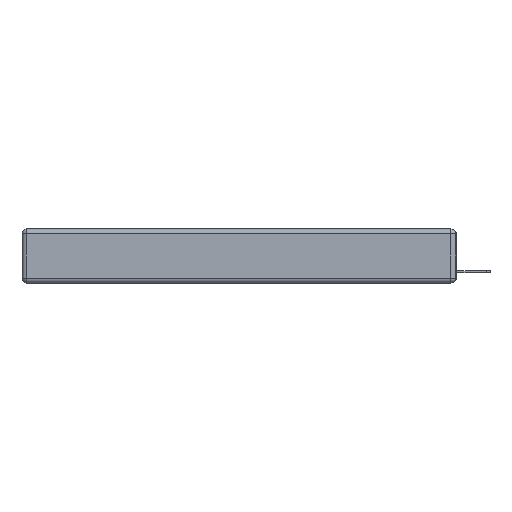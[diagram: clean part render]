
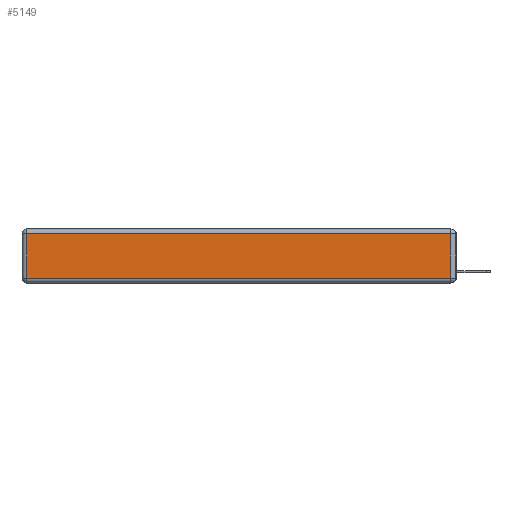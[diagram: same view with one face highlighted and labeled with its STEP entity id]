
A CAD part, left-side view. The second image highlights one B-rep face of the part: STEP entity #5149.
In plain terms, the highlighted planar face has unit normal (-1, 0, 0).
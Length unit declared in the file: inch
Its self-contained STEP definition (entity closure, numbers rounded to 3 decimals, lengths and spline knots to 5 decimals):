
#2 = VERTEX_POINT ( 'NONE', #13605 ) ;
#701 = ORIENTED_EDGE ( 'NONE', *, *, #10102, .T. ) ;
#773 = EDGE_CURVE ( 'NONE', #2, #13497, #12182, .T. ) ;
#1738 = LINE ( 'NONE', #10577, #10507 ) ;
#2370 = PLANE ( 'NONE',  #8723 ) ;
#4231 = EDGE_CURVE ( 'NONE', #13497, #7514, #11881, .T. ) ;
#4728 = CARTESIAN_POINT ( 'NONE',  ( 0., 0.03, -0.03 ) ) ;
#5092 = DIRECTION ( 'NONE',  ( 0., 0., 1. ) ) ;
#5149 = ADVANCED_FACE ( 'NONE', ( #8542 ), #2370, .T. ) ;
#5228 = CARTESIAN_POINT ( 'NONE',  ( 0., 0.03, -0.343 ) ) ;
#5507 = VECTOR ( 'NONE', #11493, 39.37008 ) ;
#5566 = VECTOR ( 'NONE', #5092, 39.37008 ) ;
#5637 = EDGE_CURVE ( 'NONE', #7514, #12082, #9065, .T. ) ;
#5860 = DIRECTION ( 'NONE',  ( -1., 0., 0. ) ) ;
#6449 = CARTESIAN_POINT ( 'NONE',  ( 0., 2.72, -0.03 ) ) ;
#7271 = ORIENTED_EDGE ( 'NONE', *, *, #5637, .T. ) ;
#7514 = VERTEX_POINT ( 'NONE', #4728 ) ;
#8079 = CARTESIAN_POINT ( 'NONE',  ( 0., 0., -0.343 ) ) ;
#8484 = DIRECTION ( 'NONE',  ( 0., 0., -1. ) ) ;
#8542 = FACE_OUTER_BOUND ( 'NONE', #14193, .T. ) ;
#8723 = AXIS2_PLACEMENT_3D ( 'NONE', #8079, #5860, #10326 ) ;
#9065 = LINE ( 'NONE', #12629, #9738 ) ;
#9738 = VECTOR ( 'NONE', #11681, 39.37008 ) ;
#10102 = EDGE_CURVE ( 'NONE', #12082, #2, #1738, .T. ) ;
#10326 = DIRECTION ( 'NONE',  ( 0., 0., 1. ) ) ;
#10507 = VECTOR ( 'NONE', #8484, 39.37008 ) ;
#10577 = CARTESIAN_POINT ( 'NONE',  ( 0., 2.72, -0.343 ) ) ;
#11493 = DIRECTION ( 'NONE',  ( 0., -1., 0. ) ) ;
#11681 = DIRECTION ( 'NONE',  ( 0., 1., 0. ) ) ;
#11769 = ORIENTED_EDGE ( 'NONE', *, *, #773, .T. ) ;
#11881 = LINE ( 'NONE', #5228, #5566 ) ;
#12082 = VERTEX_POINT ( 'NONE', #6449 ) ;
#12182 = LINE ( 'NONE', #14549, #5507 ) ;
#12578 = ORIENTED_EDGE ( 'NONE', *, *, #4231, .T. ) ;
#12629 = CARTESIAN_POINT ( 'NONE',  ( 0., 2.75, -0.03 ) ) ;
#13372 = CARTESIAN_POINT ( 'NONE',  ( 0., 0.03, -0.313 ) ) ;
#13497 = VERTEX_POINT ( 'NONE', #13372 ) ;
#13605 = CARTESIAN_POINT ( 'NONE',  ( 0., 2.72, -0.313 ) ) ;
#14193 = EDGE_LOOP ( 'NONE', ( #11769, #12578, #7271, #701 ) ) ;
#14549 = CARTESIAN_POINT ( 'NONE',  ( 0., 0., -0.313 ) ) ;
